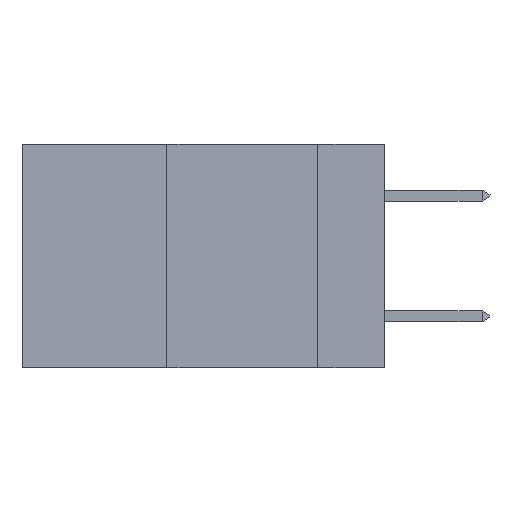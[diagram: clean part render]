
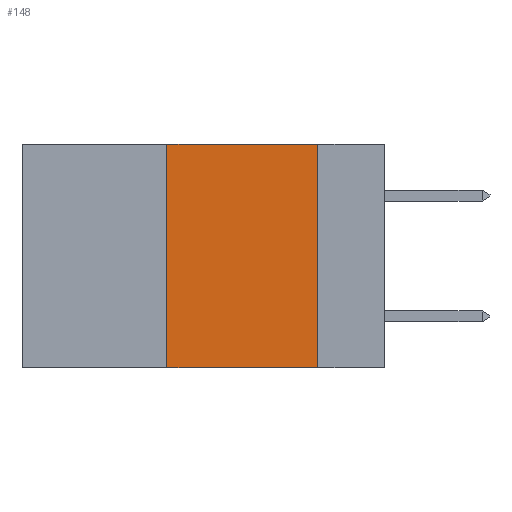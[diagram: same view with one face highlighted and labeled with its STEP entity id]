
A CAD part, left-side view. The second image highlights one B-rep face of the part: STEP entity #148.
In plain terms, the highlighted planar face has unit normal (-1, 0, 0).
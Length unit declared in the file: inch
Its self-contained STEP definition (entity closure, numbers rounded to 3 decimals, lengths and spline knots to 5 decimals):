
#148 = ADVANCED_FACE ( 'NONE', ( #16138 ), #4083, .F. ) ;
#369 = VERTEX_POINT ( 'NONE', #10404 ) ;
#1167 = LINE ( 'NONE', #12277, #13369 ) ;
#3317 = DIRECTION ( 'NONE',  ( 0., 0., -1. ) ) ;
#3993 = DIRECTION ( 'NONE',  ( 1., 0., 0. ) ) ;
#4083 = PLANE ( 'NONE',  #25768 ) ;
#4557 = CARTESIAN_POINT ( 'NONE',  ( 0., 0.36, -0.37 ) ) ;
#5408 = CARTESIAN_POINT ( 'NONE',  ( 0., 0.11, -0.37 ) ) ;
#5717 = VERTEX_POINT ( 'NONE', #4557 ) ;
#7646 = DIRECTION ( 'NONE',  ( 0., -1., 0. ) ) ;
#7709 = CARTESIAN_POINT ( 'NONE',  ( 0., 0.36, 0. ) ) ;
#7809 = ORIENTED_EDGE ( 'NONE', *, *, #8828, .F. ) ;
#8346 = CARTESIAN_POINT ( 'NONE',  ( 0., 0.6, 0. ) ) ;
#8544 = EDGE_CURVE ( 'NONE', #5717, #369, #16679, .T. ) ;
#8828 = EDGE_CURVE ( 'NONE', #13591, #11734, #10565, .T. ) ;
#9692 = DIRECTION ( 'NONE',  ( 0., 0., 1. ) ) ;
#10404 = CARTESIAN_POINT ( 'NONE',  ( 0., 0.36, 0. ) ) ;
#10565 = LINE ( 'NONE', #11614, #22771 ) ;
#10824 = CARTESIAN_POINT ( 'NONE',  ( 0., 0.11, 0. ) ) ;
#11237 = VECTOR ( 'NONE', #9692, 39.37008 ) ;
#11614 = CARTESIAN_POINT ( 'NONE',  ( 0., 0.11, 0. ) ) ;
#11734 = VERTEX_POINT ( 'NONE', #5408 ) ;
#12277 = CARTESIAN_POINT ( 'NONE',  ( 0., 0.6, 0. ) ) ;
#12677 = ORIENTED_EDGE ( 'NONE', *, *, #16071, .T. ) ;
#13369 = VECTOR ( 'NONE', #14333, 39.37008 ) ;
#13591 = VERTEX_POINT ( 'NONE', #10824 ) ;
#14333 = DIRECTION ( 'NONE',  ( 0., -1., 0. ) ) ;
#16071 = EDGE_CURVE ( 'NONE', #5717, #11734, #25229, .T. ) ;
#16138 = FACE_OUTER_BOUND ( 'NONE', #24740, .T. ) ;
#16523 = ORIENTED_EDGE ( 'NONE', *, *, #8544, .F. ) ;
#16679 = LINE ( 'NONE', #7709, #11237 ) ;
#20045 = CARTESIAN_POINT ( 'NONE',  ( 0., 0.6, -0.37 ) ) ;
#20464 = DIRECTION ( 'NONE',  ( 0., 0., -1. ) ) ;
#22771 = VECTOR ( 'NONE', #3317, 39.37008 ) ;
#24089 = EDGE_CURVE ( 'NONE', #369, #13591, #1167, .T. ) ;
#24413 = ORIENTED_EDGE ( 'NONE', *, *, #24089, .F. ) ;
#24590 = VECTOR ( 'NONE', #7646, 39.37008 ) ;
#24740 = EDGE_LOOP ( 'NONE', ( #7809, #24413, #16523, #12677 ) ) ;
#25229 = LINE ( 'NONE', #20045, #24590 ) ;
#25768 = AXIS2_PLACEMENT_3D ( 'NONE', #8346, #3993, #20464 ) ;
